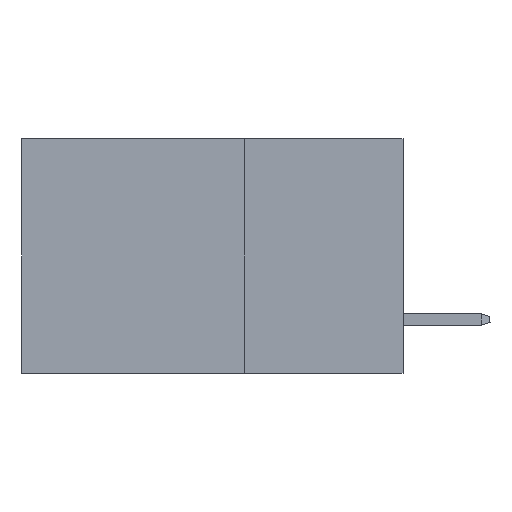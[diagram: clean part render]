
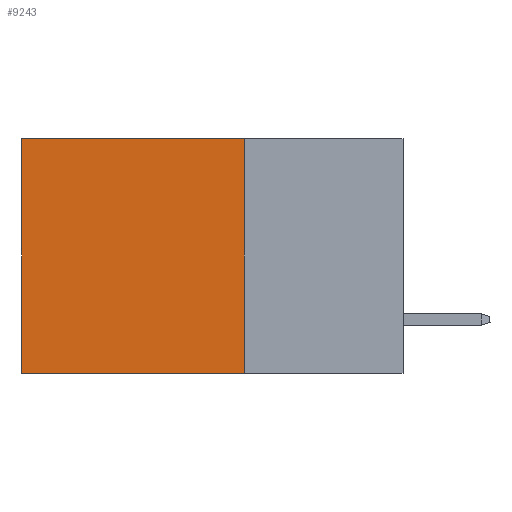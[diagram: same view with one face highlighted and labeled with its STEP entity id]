
A CAD part, left-side view. The second image highlights one B-rep face of the part: STEP entity #9243.
In plain terms, the highlighted planar face has unit normal (-1, 0, 0).
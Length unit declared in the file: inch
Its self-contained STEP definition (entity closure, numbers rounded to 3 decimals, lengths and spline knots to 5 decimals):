
#1475 = CARTESIAN_POINT ( 'NONE',  ( 0.2875, 0.6, 0. ) ) ;
#1980 = DIRECTION ( 'NONE',  ( 0., 0., -1. ) ) ;
#3233 = AXIS2_PLACEMENT_3D ( 'NONE', #23018, #17114, #7832 ) ;
#3754 = CARTESIAN_POINT ( 'NONE',  ( 0.2875, 0.25, 0. ) ) ;
#4145 = LINE ( 'NONE', #3754, #8872 ) ;
#4490 = ORIENTED_EDGE ( 'NONE', *, *, #7731, .T. ) ;
#4657 = EDGE_CURVE ( 'NONE', #14109, #8103, #6621, .T. ) ;
#4935 = CARTESIAN_POINT ( 'NONE',  ( 0.2875, 0.6, -0.37 ) ) ;
#5276 = VERTEX_POINT ( 'NONE', #1475 ) ;
#5767 = EDGE_CURVE ( 'NONE', #14109, #5276, #4145, .T. ) ;
#6464 = CARTESIAN_POINT ( 'NONE',  ( 0.2875, 0.25, -0.37 ) ) ;
#6621 = LINE ( 'NONE', #13929, #24117 ) ;
#7713 = DIRECTION ( 'NONE',  ( 0., 1., 0. ) ) ;
#7731 = EDGE_CURVE ( 'NONE', #5276, #12583, #17208, .T. ) ;
#7832 = DIRECTION ( 'NONE',  ( 0., 0., -1. ) ) ;
#8103 = VERTEX_POINT ( 'NONE', #24056 ) ;
#8872 = VECTOR ( 'NONE', #7713, 39.37008 ) ;
#9243 = ADVANCED_FACE ( 'NONE', ( #9677 ), #13305, .F. ) ;
#9677 = FACE_OUTER_BOUND ( 'NONE', #14759, .T. ) ;
#10119 = DIRECTION ( 'NONE',  ( 0., 1., 0. ) ) ;
#12583 = VERTEX_POINT ( 'NONE', #4935 ) ;
#12656 = ORIENTED_EDGE ( 'NONE', *, *, #5767, .T. ) ;
#13225 = EDGE_CURVE ( 'NONE', #8103, #12583, #19531, .T. ) ;
#13272 = CARTESIAN_POINT ( 'NONE',  ( 0.2875, 0.6, 0. ) ) ;
#13305 = PLANE ( 'NONE',  #3233 ) ;
#13929 = CARTESIAN_POINT ( 'NONE',  ( 0.2875, 0.25, 0. ) ) ;
#14027 = VECTOR ( 'NONE', #10119, 39.37008 ) ;
#14109 = VERTEX_POINT ( 'NONE', #23506 ) ;
#14759 = EDGE_LOOP ( 'NONE', ( #4490, #19829, #20169, #12656 ) ) ;
#17114 = DIRECTION ( 'NONE',  ( 1., 0., 0. ) ) ;
#17208 = LINE ( 'NONE', #13272, #23859 ) ;
#19531 = LINE ( 'NONE', #6464, #14027 ) ;
#19829 = ORIENTED_EDGE ( 'NONE', *, *, #13225, .F. ) ;
#20169 = ORIENTED_EDGE ( 'NONE', *, *, #4657, .F. ) ;
#21539 = DIRECTION ( 'NONE',  ( 0., 0., -1. ) ) ;
#23018 = CARTESIAN_POINT ( 'NONE',  ( 0.2875, 0.25, 0. ) ) ;
#23506 = CARTESIAN_POINT ( 'NONE',  ( 0.2875, 0.25, 0. ) ) ;
#23859 = VECTOR ( 'NONE', #1980, 39.37008 ) ;
#24056 = CARTESIAN_POINT ( 'NONE',  ( 0.2875, 0.25, -0.37 ) ) ;
#24117 = VECTOR ( 'NONE', #21539, 39.37008 ) ;
